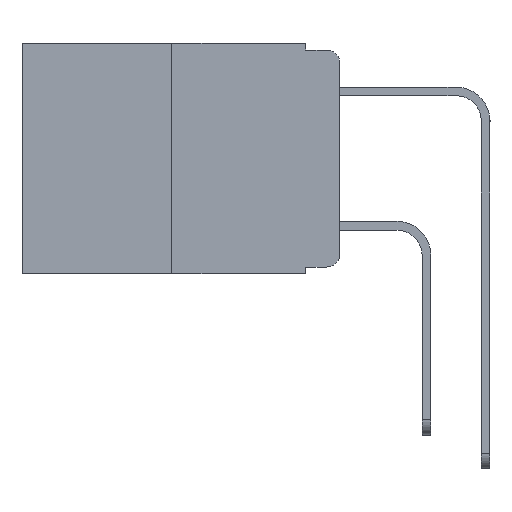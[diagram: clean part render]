
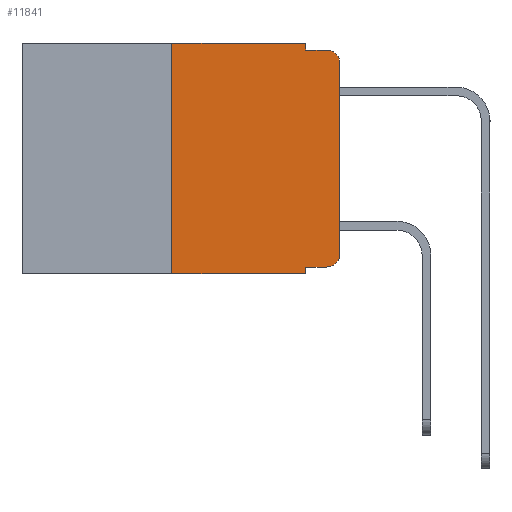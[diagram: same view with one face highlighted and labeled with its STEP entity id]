
A CAD part, left-side view. The second image highlights one B-rep face of the part: STEP entity #11841.
In plain terms, the highlighted planar face has unit normal (-1, 0, 0).
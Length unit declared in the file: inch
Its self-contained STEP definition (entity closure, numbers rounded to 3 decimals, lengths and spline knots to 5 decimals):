
#180 = DIRECTION ( 'NONE',  ( 0., -1., 0. ) ) ;
#414 = VERTEX_POINT ( 'NONE', #7816 ) ;
#416 = DIRECTION ( 'NONE',  ( 0., 0., -1. ) ) ;
#539 = EDGE_CURVE ( 'NONE', #2751, #12867, #5452, .T. ) ;
#748 = ORIENTED_EDGE ( 'NONE', *, *, #7473, .T. ) ;
#826 = LINE ( 'NONE', #12577, #11531 ) ;
#976 = DIRECTION ( 'NONE',  ( 0., 0., -1. ) ) ;
#1096 = EDGE_CURVE ( 'NONE', #414, #2751, #4968, .T. ) ;
#1244 = VERTEX_POINT ( 'NONE', #10851 ) ;
#1483 = ORIENTED_EDGE ( 'NONE', *, *, #1096, .T. ) ;
#1683 = EDGE_LOOP ( 'NONE', ( #2421, #13150, #3119, #3455, #4483, #7343, #8120, #5110, #748, #1483 ) ) ;
#1882 = VERTEX_POINT ( 'NONE', #9143 ) ;
#2017 = AXIS2_PLACEMENT_3D ( 'NONE', #9830, #3754, #10829 ) ;
#2169 = LINE ( 'NONE', #13118, #8019 ) ;
#2175 = CARTESIAN_POINT ( 'NONE',  ( 0., 0., -0.313 ) ) ;
#2186 = VERTEX_POINT ( 'NONE', #2979 ) ;
#2373 = CARTESIAN_POINT ( 'NONE',  ( 0., 0.051, -0.01 ) ) ;
#2421 = ORIENTED_EDGE ( 'NONE', *, *, #539, .T. ) ;
#2533 = VERTEX_POINT ( 'NONE', #10114 ) ;
#2751 = VERTEX_POINT ( 'NONE', #2175 ) ;
#2811 = VERTEX_POINT ( 'NONE', #4853 ) ;
#2891 = AXIS2_PLACEMENT_3D ( 'NONE', #12773, #6810, #416 ) ;
#2979 = CARTESIAN_POINT ( 'NONE',  ( 0., 0.051, -0.01 ) ) ;
#2991 = CARTESIAN_POINT ( 'NONE',  ( 0., 0., -0.03 ) ) ;
#3119 = ORIENTED_EDGE ( 'NONE', *, *, #5844, .F. ) ;
#3147 = DIRECTION ( 'NONE',  ( 0., 0., -1. ) ) ;
#3282 = CARTESIAN_POINT ( 'NONE',  ( 0., 0.051, 0. ) ) ;
#3303 = LINE ( 'NONE', #8318, #3634 ) ;
#3455 = ORIENTED_EDGE ( 'NONE', *, *, #3797, .F. ) ;
#3607 = LINE ( 'NONE', #5827, #11038 ) ;
#3634 = VECTOR ( 'NONE', #976, 39.37008 ) ;
#3754 = DIRECTION ( 'NONE',  ( -1., 0., 0. ) ) ;
#3781 = DIRECTION ( 'NONE',  ( 0., -1., 0. ) ) ;
#3797 = EDGE_CURVE ( 'NONE', #11138, #2186, #3303, .T. ) ;
#3972 = EDGE_CURVE ( 'NONE', #2533, #1244, #826, .T. ) ;
#4053 = VECTOR ( 'NONE', #9561, 39.37008 ) ;
#4276 = DIRECTION ( 'NONE',  ( 0., 0., 1. ) ) ;
#4483 = ORIENTED_EDGE ( 'NONE', *, *, #11861, .F. ) ;
#4758 = PLANE ( 'NONE',  #2891 ) ;
#4853 = CARTESIAN_POINT ( 'NONE',  ( 0., 0.051, -0.333 ) ) ;
#4968 = CIRCLE ( 'NONE', #12849, 0.02 ) ;
#5110 = ORIENTED_EDGE ( 'NONE', *, *, #9485, .F. ) ;
#5449 = CARTESIAN_POINT ( 'NONE',  ( 0., 0.02, -0.01 ) ) ;
#5452 = LINE ( 'NONE', #8930, #10494 ) ;
#5800 = VERTEX_POINT ( 'NONE', #5449 ) ;
#5827 = CARTESIAN_POINT ( 'NONE',  ( 0., 0.473, 0. ) ) ;
#5844 = EDGE_CURVE ( 'NONE', #2186, #5800, #12069, .T. ) ;
#5992 = FACE_OUTER_BOUND ( 'NONE', #1683, .T. ) ;
#6267 = DIRECTION ( 'NONE',  ( -1., 0., 0. ) ) ;
#6810 = DIRECTION ( 'NONE',  ( 1., 0., 0. ) ) ;
#7137 = CARTESIAN_POINT ( 'NONE',  ( 0., 0.02, -0.313 ) ) ;
#7201 = DIRECTION ( 'NONE',  ( 0., -1., 0. ) ) ;
#7343 = ORIENTED_EDGE ( 'NONE', *, *, #11495, .F. ) ;
#7473 = EDGE_CURVE ( 'NONE', #2811, #414, #2169, .T. ) ;
#7816 = CARTESIAN_POINT ( 'NONE',  ( 0., 0.02, -0.333 ) ) ;
#7906 = EDGE_CURVE ( 'NONE', #12867, #5800, #8606, .T. ) ;
#8019 = VECTOR ( 'NONE', #7201, 39.37008 ) ;
#8120 = ORIENTED_EDGE ( 'NONE', *, *, #3972, .T. ) ;
#8318 = CARTESIAN_POINT ( 'NONE',  ( 0., 0.051, 0. ) ) ;
#8356 = DIRECTION ( 'NONE',  ( 0., 0., -1. ) ) ;
#8606 = CIRCLE ( 'NONE', #2017, 0.02 ) ;
#8723 = VECTOR ( 'NONE', #8356, 39.37008 ) ;
#8793 = CARTESIAN_POINT ( 'NONE',  ( 0., 0.051, 0. ) ) ;
#8930 = CARTESIAN_POINT ( 'NONE',  ( 0., 0., 0. ) ) ;
#9143 = CARTESIAN_POINT ( 'NONE',  ( 0., 0.25, 0. ) ) ;
#9485 = EDGE_CURVE ( 'NONE', #2811, #1244, #11403, .T. ) ;
#9561 = DIRECTION ( 'NONE',  ( 0., -1., 0. ) ) ;
#9610 = DIRECTION ( 'NONE',  ( 0., 0., 1. ) ) ;
#9830 = CARTESIAN_POINT ( 'NONE',  ( 0., 0.02, -0.03 ) ) ;
#10114 = CARTESIAN_POINT ( 'NONE',  ( 0., 0.25, -0.343 ) ) ;
#10419 = LINE ( 'NONE', #12302, #12416 ) ;
#10494 = VECTOR ( 'NONE', #9610, 39.37008 ) ;
#10829 = DIRECTION ( 'NONE',  ( 0., 0., -1. ) ) ;
#10851 = CARTESIAN_POINT ( 'NONE',  ( 0., 0.051, -0.343 ) ) ;
#11038 = VECTOR ( 'NONE', #3781, 39.37008 ) ;
#11138 = VERTEX_POINT ( 'NONE', #8793 ) ;
#11403 = LINE ( 'NONE', #3282, #8723 ) ;
#11495 = EDGE_CURVE ( 'NONE', #2533, #1882, #10419, .T. ) ;
#11531 = VECTOR ( 'NONE', #180, 39.37008 ) ;
#11841 = ADVANCED_FACE ( 'NONE', ( #5992 ), #4758, .F. ) ;
#11861 = EDGE_CURVE ( 'NONE', #1882, #11138, #3607, .T. ) ;
#12069 = LINE ( 'NONE', #2373, #4053 ) ;
#12302 = CARTESIAN_POINT ( 'NONE',  ( 0., 0.25, 0. ) ) ;
#12416 = VECTOR ( 'NONE', #4276, 39.37008 ) ;
#12577 = CARTESIAN_POINT ( 'NONE',  ( 0., 0.473, -0.343 ) ) ;
#12773 = CARTESIAN_POINT ( 'NONE',  ( 0., 0.473, 0. ) ) ;
#12849 = AXIS2_PLACEMENT_3D ( 'NONE', #7137, #6267, #3147 ) ;
#12867 = VERTEX_POINT ( 'NONE', #2991 ) ;
#13118 = CARTESIAN_POINT ( 'NONE',  ( 0., 0.051, -0.333 ) ) ;
#13150 = ORIENTED_EDGE ( 'NONE', *, *, #7906, .T. ) ;
